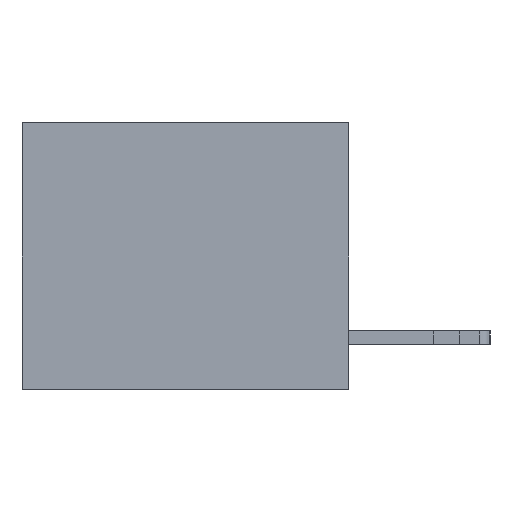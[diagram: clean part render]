
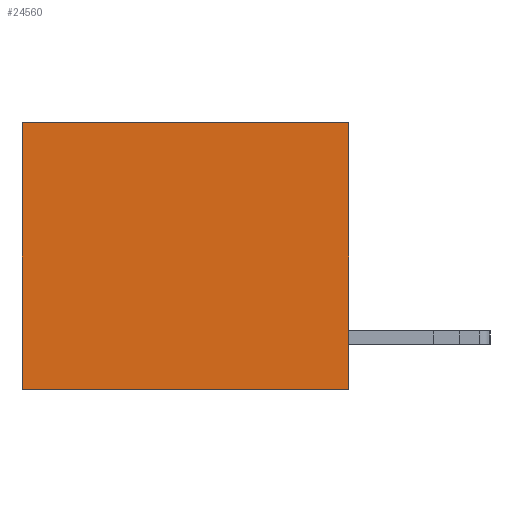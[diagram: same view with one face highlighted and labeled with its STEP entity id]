
A CAD part, left-side view. The second image highlights one B-rep face of the part: STEP entity #24560.
In plain terms, the highlighted planar face has unit normal (-1, 0, 0).
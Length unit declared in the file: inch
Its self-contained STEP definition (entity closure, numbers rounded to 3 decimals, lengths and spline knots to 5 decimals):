
#232 = VERTEX_POINT ( 'NONE', #6345 ) ;
#622 = VERTEX_POINT ( 'NONE', #7054 ) ;
#1746 = EDGE_CURVE ( 'NONE', #22013, #622, #17430, .T. ) ;
#1768 = DIRECTION ( 'NONE',  ( 0., 0., -1. ) ) ;
#1935 = CARTESIAN_POINT ( 'NONE',  ( 0.3165, 0., -0.49 ) ) ;
#2030 = DIRECTION ( 'NONE',  ( 0., 1., 0. ) ) ;
#2959 = LINE ( 'NONE', #1935, #6486 ) ;
#3776 = VERTEX_POINT ( 'NONE', #23935 ) ;
#3974 = EDGE_CURVE ( 'NONE', #22013, #232, #5530, .T. ) ;
#4736 = VECTOR ( 'NONE', #22415, 39.37008 ) ;
#5530 = LINE ( 'NONE', #20567, #9738 ) ;
#6345 = CARTESIAN_POINT ( 'NONE',  ( 0.3165, 0., -0.49 ) ) ;
#6486 = VECTOR ( 'NONE', #2030, 39.37008 ) ;
#7054 = CARTESIAN_POINT ( 'NONE',  ( 0.3165, 0.6, 0. ) ) ;
#8714 = CARTESIAN_POINT ( 'NONE',  ( 0.3165, 0., 0. ) ) ;
#9738 = VECTOR ( 'NONE', #26626, 39.37008 ) ;
#10271 = ORIENTED_EDGE ( 'NONE', *, *, #1746, .T. ) ;
#11245 = EDGE_LOOP ( 'NONE', ( #23977, #21419, #25836, #10271 ) ) ;
#11485 = EDGE_CURVE ( 'NONE', #622, #3776, #17019, .T. ) ;
#13545 = AXIS2_PLACEMENT_3D ( 'NONE', #14091, #16343, #1768 ) ;
#14091 = CARTESIAN_POINT ( 'NONE',  ( 0.3165, 0., -0.49 ) ) ;
#14878 = VECTOR ( 'NONE', #22829, 39.37008 ) ;
#16343 = DIRECTION ( 'NONE',  ( 1., 0., 0. ) ) ;
#16840 = EDGE_CURVE ( 'NONE', #232, #3776, #2959, .T. ) ;
#16969 = CARTESIAN_POINT ( 'NONE',  ( 0.3165, 0., 0. ) ) ;
#17019 = LINE ( 'NONE', #20049, #4736 ) ;
#17430 = LINE ( 'NONE', #8714, #14878 ) ;
#20049 = CARTESIAN_POINT ( 'NONE',  ( 0.3165, 0.6, -0.49 ) ) ;
#20096 = PLANE ( 'NONE',  #13545 ) ;
#20567 = CARTESIAN_POINT ( 'NONE',  ( 0.3165, 0., -0.49 ) ) ;
#21419 = ORIENTED_EDGE ( 'NONE', *, *, #16840, .F. ) ;
#22013 = VERTEX_POINT ( 'NONE', #16969 ) ;
#22415 = DIRECTION ( 'NONE',  ( 0., 0., -1. ) ) ;
#22829 = DIRECTION ( 'NONE',  ( 0., 1., 0. ) ) ;
#23935 = CARTESIAN_POINT ( 'NONE',  ( 0.3165, 0.6, -0.49 ) ) ;
#23977 = ORIENTED_EDGE ( 'NONE', *, *, #11485, .T. ) ;
#24560 = ADVANCED_FACE ( 'NONE', ( #26699 ), #20096, .F. ) ;
#25836 = ORIENTED_EDGE ( 'NONE', *, *, #3974, .F. ) ;
#26626 = DIRECTION ( 'NONE',  ( 0., 0., -1. ) ) ;
#26699 = FACE_OUTER_BOUND ( 'NONE', #11245, .T. ) ;
